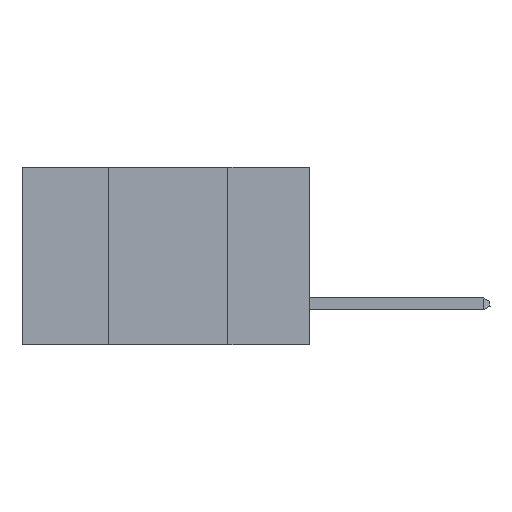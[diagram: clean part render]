
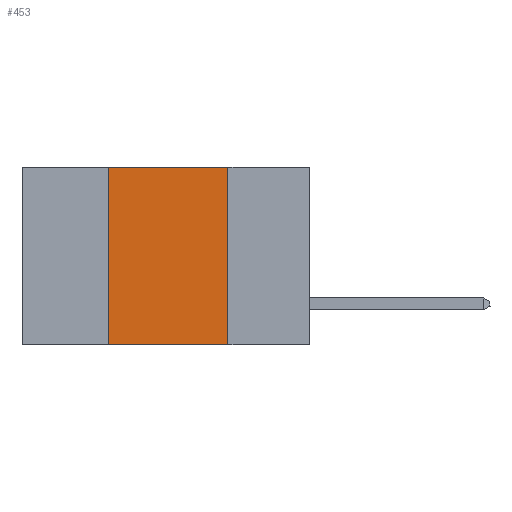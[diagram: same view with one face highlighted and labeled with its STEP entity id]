
A CAD part, left-side view. The second image highlights one B-rep face of the part: STEP entity #453.
In plain terms, the highlighted planar face has unit normal (-1, 0, 0).
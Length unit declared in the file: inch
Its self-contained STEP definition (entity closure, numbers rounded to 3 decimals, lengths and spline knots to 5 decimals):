
#206 = CARTESIAN_POINT ( 'NONE',  ( 0., 0.6, -0.37 ) ) ;
#453 = ADVANCED_FACE ( 'NONE', ( #15175 ), #7880, .F. ) ;
#501 = CARTESIAN_POINT ( 'NONE',  ( 0., 0.42, 0. ) ) ;
#915 = ORIENTED_EDGE ( 'NONE', *, *, #13626, .F. ) ;
#1126 = EDGE_CURVE ( 'NONE', #8774, #12142, #8035, .T. ) ;
#1298 = VECTOR ( 'NONE', #5282, 39.37008 ) ;
#1503 = CARTESIAN_POINT ( 'NONE',  ( 0., 0.42, -0.37 ) ) ;
#1533 = EDGE_CURVE ( 'NONE', #12134, #15801, #7056, .T. ) ;
#1540 = EDGE_LOOP ( 'NONE', ( #9396, #915, #13208, #14773 ) ) ;
#2788 = DIRECTION ( 'NONE',  ( 1., 0., 0. ) ) ;
#5282 = DIRECTION ( 'NONE',  ( 0., -1., 0. ) ) ;
#5333 = CARTESIAN_POINT ( 'NONE',  ( 0., 0.42, 0. ) ) ;
#5422 = DIRECTION ( 'NONE',  ( 0., 0., -1. ) ) ;
#5854 = DIRECTION ( 'NONE',  ( 0., -1., 0. ) ) ;
#6081 = VECTOR ( 'NONE', #5854, 39.37008 ) ;
#6178 = DIRECTION ( 'NONE',  ( 0., 0., -1. ) ) ;
#7056 = LINE ( 'NONE', #11163, #9821 ) ;
#7880 = PLANE ( 'NONE',  #11188 ) ;
#8035 = LINE ( 'NONE', #501, #14948 ) ;
#8774 = VERTEX_POINT ( 'NONE', #1503 ) ;
#8988 = CARTESIAN_POINT ( 'NONE',  ( 0., 0.6, 0. ) ) ;
#9396 = ORIENTED_EDGE ( 'NONE', *, *, #1533, .F. ) ;
#9821 = VECTOR ( 'NONE', #6178, 39.37008 ) ;
#10742 = DIRECTION ( 'NONE',  ( 0., 0., 1. ) ) ;
#10969 = CARTESIAN_POINT ( 'NONE',  ( 0., 0.17, -0.37 ) ) ;
#11163 = CARTESIAN_POINT ( 'NONE',  ( 0., 0.17, 0. ) ) ;
#11188 = AXIS2_PLACEMENT_3D ( 'NONE', #8988, #2788, #5422 ) ;
#11382 = LINE ( 'NONE', #13482, #6081 ) ;
#12134 = VERTEX_POINT ( 'NONE', #14108 ) ;
#12142 = VERTEX_POINT ( 'NONE', #5333 ) ;
#13208 = ORIENTED_EDGE ( 'NONE', *, *, #1126, .F. ) ;
#13482 = CARTESIAN_POINT ( 'NONE',  ( 0., 0.6, 0. ) ) ;
#13626 = EDGE_CURVE ( 'NONE', #12142, #12134, #11382, .T. ) ;
#14108 = CARTESIAN_POINT ( 'NONE',  ( 0., 0.17, 0. ) ) ;
#14773 = ORIENTED_EDGE ( 'NONE', *, *, #15172, .T. ) ;
#14948 = VECTOR ( 'NONE', #10742, 39.37008 ) ;
#15172 = EDGE_CURVE ( 'NONE', #8774, #15801, #15259, .T. ) ;
#15175 = FACE_OUTER_BOUND ( 'NONE', #1540, .T. ) ;
#15259 = LINE ( 'NONE', #206, #1298 ) ;
#15801 = VERTEX_POINT ( 'NONE', #10969 ) ;
